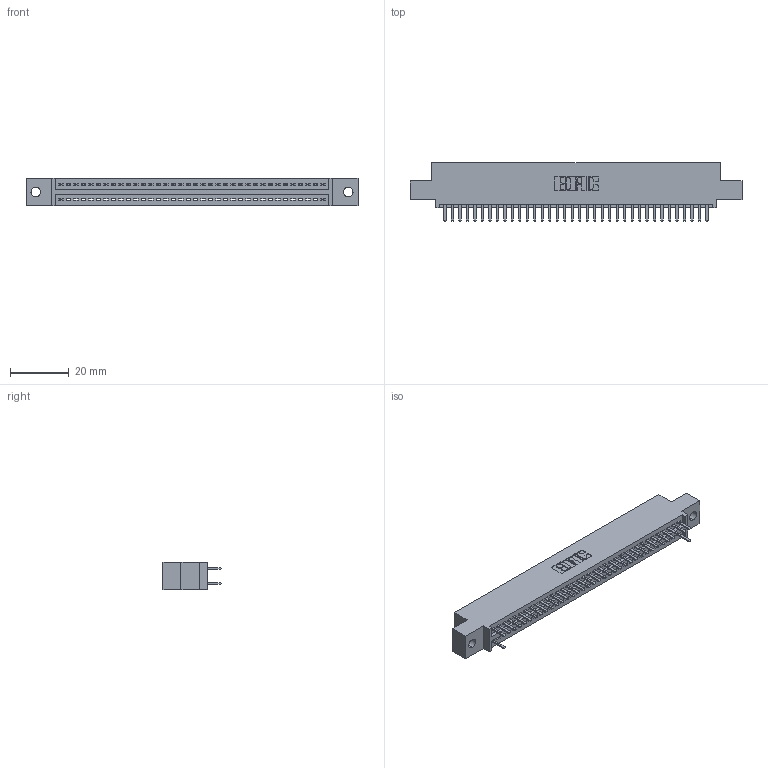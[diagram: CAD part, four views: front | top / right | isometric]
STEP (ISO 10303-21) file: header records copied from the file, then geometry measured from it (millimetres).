
FILE_DESCRIPTION (( 'STEP AP203' ), '1' );
FILE_NAME ('395-072-520-502.STEP', '2018-11-27T08:10:24', ( '' ), ( '' ), 'SwSTEP 2.0', 'SolidWorks 2016', '' );
FILE_SCHEMA (( 'CONFIG_CONTROL_DESIGN' ));
Length unit declared in the file: inch
Products named in the file (3): 395-072-520-502; 345 Part_0.110 Offset - 0.128 Dia; 345-292-001_345-293-120
Assembly tree (39 placements, depth 2):
  395-072-520-502
    345 Part_0.110 Offset - 0.128 Dia
    345-292-001_345-293-120  x38
Bounding box: 112.65 x 19.68 x 9.4 mm (x, y, z)
Volume: 10453.9 mm3; surface area: 13385.2 mm2
Topology: 39 solids, 39 shells, 2454 faces, 7237 edges, 4722 vertices
Faces by surface type: plane 1652, cylinder 802
Entity records: 28215 total; most frequent: CARTESIAN_POINT 4898, ORIENTED_EDGE 4854, DIRECTION 4275, EDGE_CURVE 2427, VECTOR 2147, LINE 2147, VERTEX_POINT 1614, AXIS2_PLACEMENT_3D 1064
